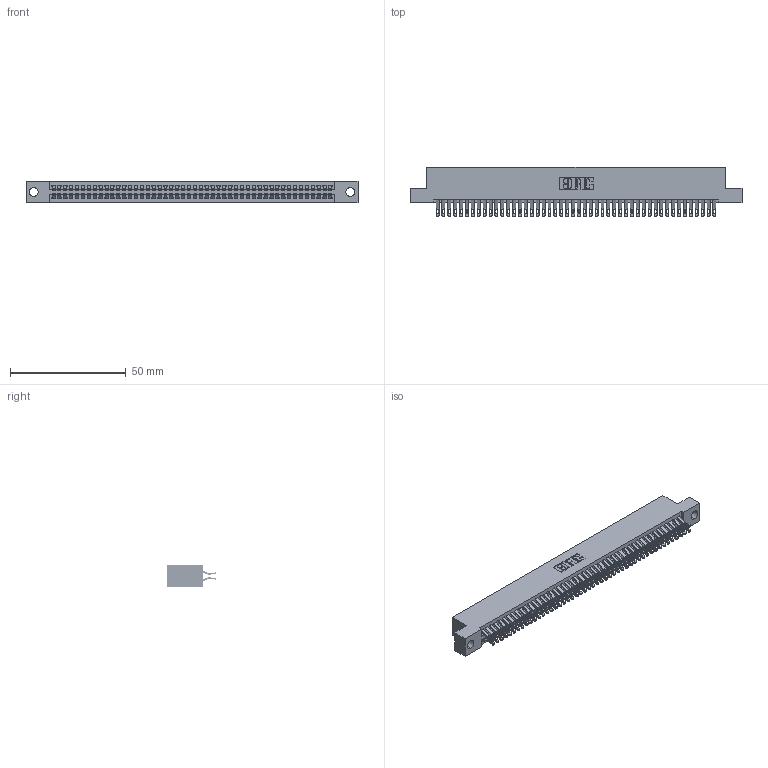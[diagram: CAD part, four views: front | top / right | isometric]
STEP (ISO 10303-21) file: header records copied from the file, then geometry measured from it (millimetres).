
FILE_DESCRIPTION (( 'STEP AP203' ), '1' );
FILE_NAME ('345-096-555-204.STEP', '2018-10-05T05:56:24', ( '' ), ( '' ), 'SwSTEP 2.0', 'SolidWorks 2016', '' );
FILE_SCHEMA (( 'CONFIG_CONTROL_DESIGN' ));
Length unit declared in the file: inch
Products named in the file (3): 345-292-001_555 Tail; 345 Part_Flush Mounting Lugs - 0.156 Dia-TH; 345-096-555-204
Assembly tree (97 placements, depth 2):
  345-096-555-204
    345 Part_Flush Mounting Lugs - 0.156 Dia-TH
    345-292-001_555 Tail  x96
Bounding box: 143.13 x 21.13 x 9.4 mm (x, y, z)
Volume: 14150 mm3; surface area: 21815.9 mm2
Topology: 97 solids, 97 shells, 5502 faces, 17333 edges, 11554 vertices
Faces by surface type: plane 3056, cylinder 2446
Entity records: 37183 total; most frequent: CARTESIAN_POINT 6262, ORIENTED_EDGE 6166, DIRECTION 5483, EDGE_CURVE 3083, LINE 2739, VECTOR 2739, VERTEX_POINT 2054, AXIS2_PLACEMENT_3D 1372
